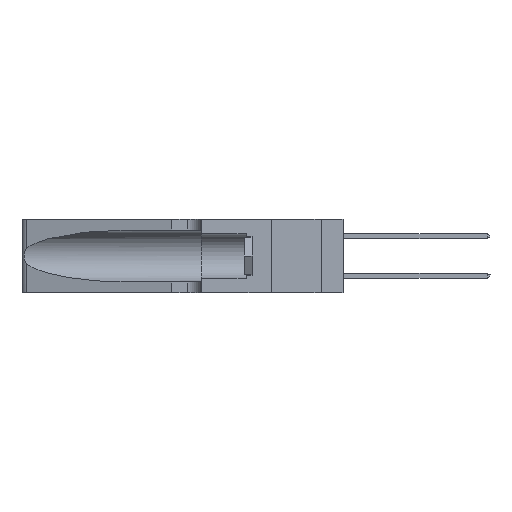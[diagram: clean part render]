
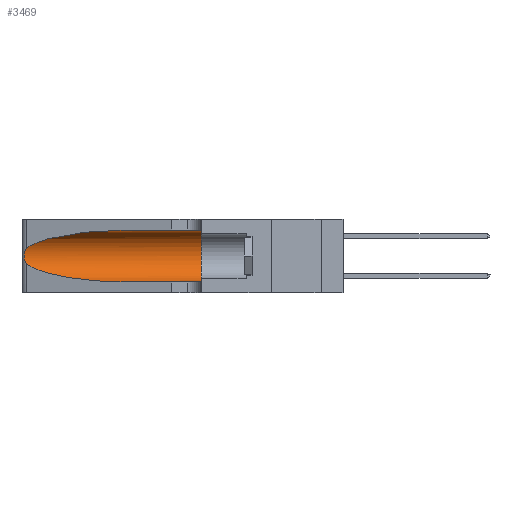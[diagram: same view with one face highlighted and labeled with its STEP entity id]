
A CAD part, left-side view. The second image highlights one B-rep face of the part: STEP entity #3469.
In plain terms, the highlighted cylindrical face has radius 3.308 mm (diameter 6.617 mm), a partial arc.
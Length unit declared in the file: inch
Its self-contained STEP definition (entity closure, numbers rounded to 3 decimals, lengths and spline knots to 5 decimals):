
#82 = DIRECTION ( 'NONE',  ( 0., 0., 1. ) ) ;
#264 = DIRECTION ( 'NONE',  ( 0., -1., 0. ) ) ;
#265 = CARTESIAN_POINT ( 'NONE',  ( 0.25487, 1.22718, 0.22369 ) ) ;
#1320 = VERTEX_POINT ( 'NONE', #15248 ) ;
#1914 = CARTESIAN_POINT ( 'NONE',  ( 0.1305, 0.35, 0.185 ) ) ;
#2398 = AXIS2_PLACEMENT_3D ( 'NONE', #15966, #2608, #20730 ) ;
#2608 = DIRECTION ( 'NONE',  ( 0., -1., 0. ) ) ;
#2928 = EDGE_CURVE ( 'NONE', #12324, #20738, #10832, .T. ) ;
#3244 = EDGE_LOOP ( 'NONE', ( #13889, #16892, #21911, #9523, #18133, #9202 ) ) ;
#3469 = ADVANCED_FACE ( 'NONE', ( #4660 ), #12028, .F. ) ;
#3487 =( BOUNDED_CURVE ( )  B_SPLINE_CURVE ( 3, ( #4100, #10747, #14560, #19062 ),
 .UNSPECIFIED., .F., .T. ) 
 B_SPLINE_CURVE_WITH_KNOTS ( ( 4, 4 ),
 ( 3.44316, 4.71239 ),
 .UNSPECIFIED. ) 
 CURVE ( )  GEOMETRIC_REPRESENTATION_ITEM ( )  RATIONAL_B_SPLINE_CURVE ( ( 1., 0.87, 0.87, 1. ) ) 
 REPRESENTATION_ITEM ( '' )  );
#4100 = CARTESIAN_POINT ( 'NONE',  ( 0.25487, 1.22718, 0.14631 ) ) ;
#4660 = FACE_OUTER_BOUND ( 'NONE', #3244, .T. ) ;
#6228 = VERTEX_POINT ( 'NONE', #11599 ) ;
#6845 = CARTESIAN_POINT ( 'NONE',  ( 0.25555, 1.22994, 0.2215 ) ) ;
#7003 = CARTESIAN_POINT ( 'NONE',  ( 0.25487, 1.22718, 0.22369 ) ) ;
#8681 = B_SPLINE_CURVE_WITH_KNOTS ( 'NONE', 3,
 ( #265, #6845, #20041, #22536, #27009, #15931, #11927, #9472, #27595, #11647, #27206, #16133, #18867, #12214 ),
 .UNSPECIFIED., .F., .F.,
 ( 4, 2, 2, 2, 2, 2, 4 ),
 ( 0., 0.00027, 0.00053, 0.00107, 0.0016, 0.00187, 0.00214 ),
 .UNSPECIFIED. ) ;
#9202 = ORIENTED_EDGE ( 'NONE', *, *, #16859, .F. ) ;
#9232 = EDGE_CURVE ( 'NONE', #20738, #6228, #8681, .T. ) ;
#9472 = CARTESIAN_POINT ( 'NONE',  ( 0.26075, 1.23896, 0.178 ) ) ;
#9523 = ORIENTED_EDGE ( 'NONE', *, *, #17196, .T. ) ;
#10747 = CARTESIAN_POINT ( 'NONE',  ( 0.2373, 1.15595, 0.08982 ) ) ;
#10832 =( BOUNDED_CURVE ( )  B_SPLINE_CURVE ( 3, ( #12024, #25056, #14061, #18672 ),
 .UNSPECIFIED., .F., .T. ) 
 B_SPLINE_CURVE_WITH_KNOTS ( ( 4, 4 ),
 ( 1.5708, 2.84003 ),
 .UNSPECIFIED. ) 
 CURVE ( )  GEOMETRIC_REPRESENTATION_ITEM ( )  RATIONAL_B_SPLINE_CURVE ( ( 1., 0.87, 0.87, 1. ) ) 
 REPRESENTATION_ITEM ( '' )  );
#11283 = EDGE_CURVE ( 'NONE', #6228, #1320, #3487, .T. ) ;
#11351 = CARTESIAN_POINT ( 'NONE',  ( 0.1305, 1.61858, 0.31525 ) ) ;
#11599 = CARTESIAN_POINT ( 'NONE',  ( 0.25487, 1.22718, 0.14631 ) ) ;
#11647 = CARTESIAN_POINT ( 'NONE',  ( 0.25856, 1.23593, 0.16098 ) ) ;
#11927 = CARTESIAN_POINT ( 'NONE',  ( 0.26075, 1.23896, 0.19203 ) ) ;
#12024 = CARTESIAN_POINT ( 'NONE',  ( 0.1305, 0.72297, 0.31525 ) ) ;
#12028 = CYLINDRICAL_SURFACE ( 'NONE', #2398, 0.13025 ) ;
#12214 = CARTESIAN_POINT ( 'NONE',  ( 0.25487, 1.22718, 0.14631 ) ) ;
#12324 = VERTEX_POINT ( 'NONE', #14725 ) ;
#12591 = CARTESIAN_POINT ( 'NONE',  ( 0.1305, 1.61858, 0.05475 ) ) ;
#12732 = VERTEX_POINT ( 'NONE', #21006 ) ;
#13889 = ORIENTED_EDGE ( 'NONE', *, *, #2928, .T. ) ;
#14061 = CARTESIAN_POINT ( 'NONE',  ( 0.2373, 1.15595, 0.28018 ) ) ;
#14560 = CARTESIAN_POINT ( 'NONE',  ( 0.18966, 0.96281, 0.05475 ) ) ;
#14725 = CARTESIAN_POINT ( 'NONE',  ( 0.1305, 0.72297, 0.31525 ) ) ;
#15248 = CARTESIAN_POINT ( 'NONE',  ( 0.1305, 0.72297, 0.05475 ) ) ;
#15481 = VECTOR ( 'NONE', #21388, 39.37008 ) ;
#15931 = CARTESIAN_POINT ( 'NONE',  ( 0.26018, 1.23835, 0.19895 ) ) ;
#15966 = CARTESIAN_POINT ( 'NONE',  ( 0.1305, 1.61858, 0.185 ) ) ;
#16133 = CARTESIAN_POINT ( 'NONE',  ( 0.25639, 1.23186, 0.15144 ) ) ;
#16184 = LINE ( 'NONE', #12591, #15481 ) ;
#16859 = EDGE_CURVE ( 'NONE', #12324, #23386, #18654, .T. ) ;
#16892 = ORIENTED_EDGE ( 'NONE', *, *, #9232, .T. ) ;
#17196 = EDGE_CURVE ( 'NONE', #1320, #12732, #16184, .T. ) ;
#18070 = CARTESIAN_POINT ( 'NONE',  ( 0.1305, 0.35, 0.31525 ) ) ;
#18133 = ORIENTED_EDGE ( 'NONE', *, *, #28315, .F. ) ;
#18654 = LINE ( 'NONE', #11351, #23150 ) ;
#18672 = CARTESIAN_POINT ( 'NONE',  ( 0.25487, 1.22718, 0.22369 ) ) ;
#18867 = CARTESIAN_POINT ( 'NONE',  ( 0.25555, 1.22993, 0.14849 ) ) ;
#19062 = CARTESIAN_POINT ( 'NONE',  ( 0.1305, 0.72297, 0.05475 ) ) ;
#19684 = CIRCLE ( 'NONE', #25426, 0.13025 ) ;
#20041 = CARTESIAN_POINT ( 'NONE',  ( 0.25639, 1.23184, 0.21858 ) ) ;
#20730 = DIRECTION ( 'NONE',  ( 0., 0., -1. ) ) ;
#20738 = VERTEX_POINT ( 'NONE', #7003 ) ;
#21006 = CARTESIAN_POINT ( 'NONE',  ( 0.1305, 0.35, 0.05475 ) ) ;
#21388 = DIRECTION ( 'NONE',  ( 0., -1., 0. ) ) ;
#21911 = ORIENTED_EDGE ( 'NONE', *, *, #11283, .T. ) ;
#22536 = CARTESIAN_POINT ( 'NONE',  ( 0.25787, 1.23484, 0.2124 ) ) ;
#23150 = VECTOR ( 'NONE', #264, 39.37008 ) ;
#23386 = VERTEX_POINT ( 'NONE', #18070 ) ;
#24304 = DIRECTION ( 'NONE',  ( 0., 1., 0. ) ) ;
#25056 = CARTESIAN_POINT ( 'NONE',  ( 0.18966, 0.96281, 0.31525 ) ) ;
#25426 = AXIS2_PLACEMENT_3D ( 'NONE', #1914, #24304, #82 ) ;
#27009 = CARTESIAN_POINT ( 'NONE',  ( 0.25854, 1.2359, 0.20912 ) ) ;
#27206 = CARTESIAN_POINT ( 'NONE',  ( 0.25789, 1.23486, 0.15765 ) ) ;
#27595 = CARTESIAN_POINT ( 'NONE',  ( 0.26017, 1.23833, 0.17102 ) ) ;
#28315 = EDGE_CURVE ( 'NONE', #23386, #12732, #19684, .T. ) ;
